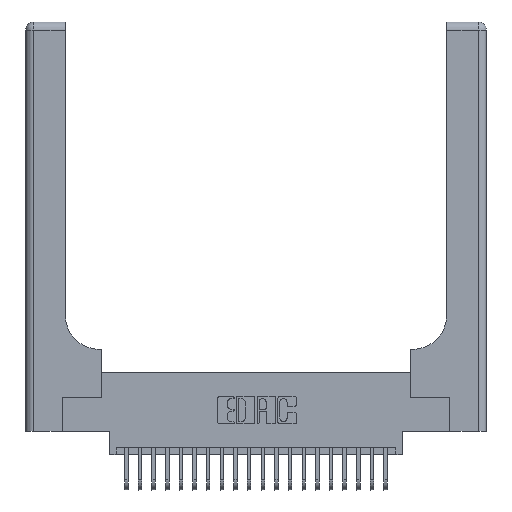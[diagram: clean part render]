
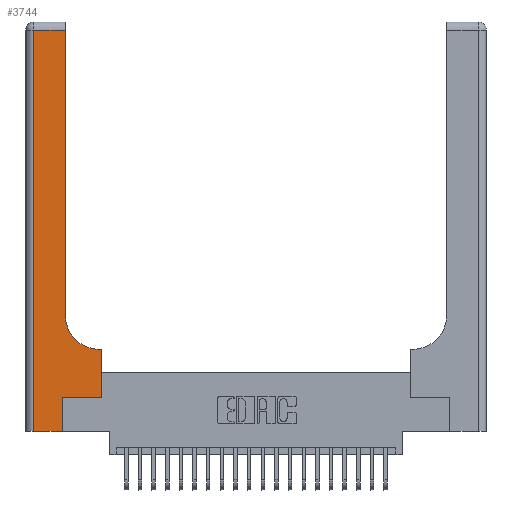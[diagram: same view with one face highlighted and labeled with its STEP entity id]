
A CAD part, top view. The second image highlights one B-rep face of the part: STEP entity #3744.
In plain terms, the highlighted planar face has unit normal (0, 0, 1).
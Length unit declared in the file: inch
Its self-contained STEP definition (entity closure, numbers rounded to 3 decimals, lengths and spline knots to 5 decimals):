
#338 = DIRECTION ( 'NONE',  ( 0., 1., 0. ) ) ;
#468 = LINE ( 'NONE', #15754, #9694 ) ;
#1038 = EDGE_CURVE ( 'NONE', #1568, #21759, #15960, .T. ) ;
#1110 = EDGE_CURVE ( 'NONE', #21759, #11856, #10065, .T. ) ;
#1475 = VECTOR ( 'NONE', #16508, 39.37008 ) ;
#1568 = VERTEX_POINT ( 'NONE', #9297 ) ;
#2611 = ORIENTED_EDGE ( 'NONE', *, *, #1038, .T. ) ;
#2816 = EDGE_CURVE ( 'NONE', #18207, #16617, #9173, .T. ) ;
#3199 = ORIENTED_EDGE ( 'NONE', *, *, #19237, .T. ) ;
#3208 = CARTESIAN_POINT ( 'NONE',  ( 0.06, 3., 0.37 ) ) ;
#3406 = CARTESIAN_POINT ( 'NONE',  ( 0.2915, 2.94, 0.37 ) ) ;
#3744 = ADVANCED_FACE ( 'NONE', ( #16451 ), #10797, .F. ) ;
#3967 = DIRECTION ( 'NONE',  ( 0., 1., 0. ) ) ;
#4570 = DIRECTION ( 'NONE',  ( 0., 1., 0. ) ) ;
#5526 = VERTEX_POINT ( 'NONE', #6843 ) ;
#5805 = CARTESIAN_POINT ( 'NONE',  ( 0.269, 0.25, 0.37 ) ) ;
#6145 = LINE ( 'NONE', #12936, #10312 ) ;
#6399 = EDGE_CURVE ( 'NONE', #20106, #22137, #468, .T. ) ;
#6843 = CARTESIAN_POINT ( 'NONE',  ( 0.06, 0., 0.37 ) ) ;
#7250 = CARTESIAN_POINT ( 'NONE',  ( 0., 3., 0.37 ) ) ;
#7588 = CARTESIAN_POINT ( 'NONE',  ( 0.5585, 0.25, 0.37 ) ) ;
#8928 = CARTESIAN_POINT ( 'NONE',  ( 0.5415, 0.85, 0.37 ) ) ;
#9087 = VECTOR ( 'NONE', #22929, 39.37008 ) ;
#9173 = CIRCLE ( 'NONE', #20675, 0.25 ) ;
#9297 = CARTESIAN_POINT ( 'NONE',  ( 0.269, 0.25, 0.37 ) ) ;
#9644 = DIRECTION ( 'NONE',  ( 1., 0., 0. ) ) ;
#9654 = LINE ( 'NONE', #3208, #9087 ) ;
#9694 = VECTOR ( 'NONE', #17537, 39.37008 ) ;
#10065 = LINE ( 'NONE', #11349, #14265 ) ;
#10312 = VECTOR ( 'NONE', #3967, 39.37008 ) ;
#10699 = EDGE_CURVE ( 'NONE', #16617, #20106, #16814, .T. ) ;
#10725 = DIRECTION ( 'NONE',  ( 1., 0., 0. ) ) ;
#10797 = PLANE ( 'NONE',  #15812 ) ;
#11349 = CARTESIAN_POINT ( 'NONE',  ( 0.5585, 0.25, 0.37 ) ) ;
#11856 = VERTEX_POINT ( 'NONE', #12297 ) ;
#12064 = EDGE_CURVE ( 'NONE', #23132, #1568, #6145, .T. ) ;
#12172 = EDGE_CURVE ( 'NONE', #5526, #23132, #18133, .T. ) ;
#12290 = CARTESIAN_POINT ( 'NONE',  ( 0.06, 2.94, 0.37 ) ) ;
#12297 = CARTESIAN_POINT ( 'NONE',  ( 0.5585, 0.6, 0.37 ) ) ;
#12598 = DIRECTION ( 'NONE',  ( -1., 0., 0. ) ) ;
#12636 = VECTOR ( 'NONE', #4570, 39.37008 ) ;
#12936 = CARTESIAN_POINT ( 'NONE',  ( 0.269, 0., 0.37 ) ) ;
#13090 = ORIENTED_EDGE ( 'NONE', *, *, #10699, .T. ) ;
#13919 = ORIENTED_EDGE ( 'NONE', *, *, #2816, .T. ) ;
#14189 = ORIENTED_EDGE ( 'NONE', *, *, #12172, .T. ) ;
#14265 = VECTOR ( 'NONE', #338, 39.37008 ) ;
#14375 = LINE ( 'NONE', #17029, #23272 ) ;
#15596 = EDGE_LOOP ( 'NONE', ( #13090, #22517, #23081, #14189, #20583, #2611, #16997, #3199, #13919 ) ) ;
#15754 = CARTESIAN_POINT ( 'NONE',  ( 0., 2.94, 0.37 ) ) ;
#15812 = AXIS2_PLACEMENT_3D ( 'NONE', #7250, #23251, #12598 ) ;
#15960 = LINE ( 'NONE', #5805, #1475 ) ;
#16451 = FACE_OUTER_BOUND ( 'NONE', #15596, .T. ) ;
#16508 = DIRECTION ( 'NONE',  ( 1., 0., 0. ) ) ;
#16617 = VERTEX_POINT ( 'NONE', #20250 ) ;
#16752 = CARTESIAN_POINT ( 'NONE',  ( 0., 0., 0.37 ) ) ;
#16814 = LINE ( 'NONE', #20637, #12636 ) ;
#16997 = ORIENTED_EDGE ( 'NONE', *, *, #1110, .T. ) ;
#17029 = CARTESIAN_POINT ( 'NONE',  ( 0.2915, 0.6, 0.37 ) ) ;
#17537 = DIRECTION ( 'NONE',  ( -1., 0., 0. ) ) ;
#18133 = LINE ( 'NONE', #16752, #22274 ) ;
#18207 = VERTEX_POINT ( 'NONE', #23042 ) ;
#18785 = EDGE_CURVE ( 'NONE', #22137, #5526, #9654, .T. ) ;
#18804 = DIRECTION ( 'NONE',  ( -1., 0., 0. ) ) ;
#18916 = CARTESIAN_POINT ( 'NONE',  ( 0.269, 0., 0.37 ) ) ;
#19237 = EDGE_CURVE ( 'NONE', #11856, #18207, #14375, .T. ) ;
#20106 = VERTEX_POINT ( 'NONE', #3406 ) ;
#20250 = CARTESIAN_POINT ( 'NONE',  ( 0.2915, 0.85, 0.37 ) ) ;
#20583 = ORIENTED_EDGE ( 'NONE', *, *, #12064, .T. ) ;
#20637 = CARTESIAN_POINT ( 'NONE',  ( 0.2915, 3., 0.37 ) ) ;
#20675 = AXIS2_PLACEMENT_3D ( 'NONE', #8928, #21376, #10725 ) ;
#21376 = DIRECTION ( 'NONE',  ( 0., 0., -1. ) ) ;
#21759 = VERTEX_POINT ( 'NONE', #7588 ) ;
#22137 = VERTEX_POINT ( 'NONE', #12290 ) ;
#22274 = VECTOR ( 'NONE', #9644, 39.37008 ) ;
#22517 = ORIENTED_EDGE ( 'NONE', *, *, #6399, .T. ) ;
#22929 = DIRECTION ( 'NONE',  ( 0., -1., 0. ) ) ;
#23042 = CARTESIAN_POINT ( 'NONE',  ( 0.5415, 0.6, 0.37 ) ) ;
#23081 = ORIENTED_EDGE ( 'NONE', *, *, #18785, .T. ) ;
#23132 = VERTEX_POINT ( 'NONE', #18916 ) ;
#23251 = DIRECTION ( 'NONE',  ( 0., 0., -1. ) ) ;
#23272 = VECTOR ( 'NONE', #18804, 39.37008 ) ;
